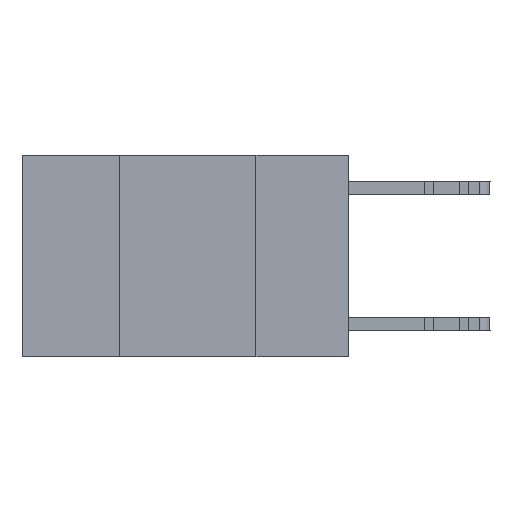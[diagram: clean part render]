
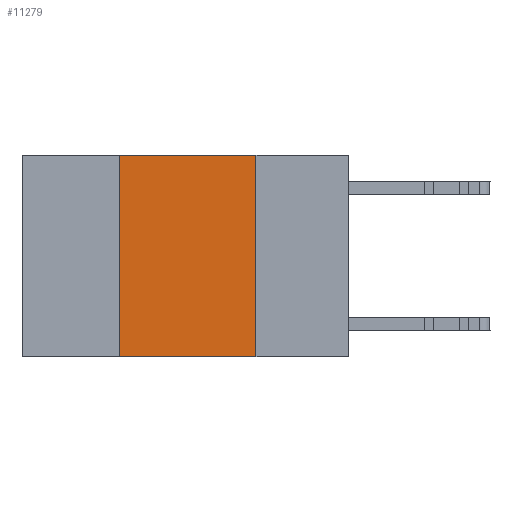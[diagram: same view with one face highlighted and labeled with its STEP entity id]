
A CAD part, left-side view. The second image highlights one B-rep face of the part: STEP entity #11279.
In plain terms, the highlighted planar face has unit normal (-1, 0, 0).
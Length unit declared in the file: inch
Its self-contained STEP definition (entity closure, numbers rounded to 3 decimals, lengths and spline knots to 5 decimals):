
#52 = AXIS2_PLACEMENT_3D ( 'NONE', #11438, #1802, #20183 ) ;
#562 = CARTESIAN_POINT ( 'NONE',  ( 0., 0.42, 0. ) ) ;
#813 = VERTEX_POINT ( 'NONE', #562 ) ;
#1142 = VERTEX_POINT ( 'NONE', #29963 ) ;
#1186 = DIRECTION ( 'NONE',  ( 0., 0., -1. ) ) ;
#1802 = DIRECTION ( 'NONE',  ( 1., 0., 0. ) ) ;
#2412 = DIRECTION ( 'NONE',  ( 0., -1., 0. ) ) ;
#3195 = LINE ( 'NONE', #12538, #23407 ) ;
#3553 = CARTESIAN_POINT ( 'NONE',  ( 0., 0.42, -0.37 ) ) ;
#8365 = LINE ( 'NONE', #12520, #25971 ) ;
#8498 = CARTESIAN_POINT ( 'NONE',  ( 0., 0.42, 0. ) ) ;
#9280 = ORIENTED_EDGE ( 'NONE', *, *, #28900, .T. ) ;
#11166 = EDGE_CURVE ( 'NONE', #21873, #1142, #8365, .T. ) ;
#11279 = ADVANCED_FACE ( 'NONE', ( #16219 ), #15923, .F. ) ;
#11438 = CARTESIAN_POINT ( 'NONE',  ( 0., 0.6, 0. ) ) ;
#12480 = EDGE_LOOP ( 'NONE', ( #18365, #25222, #22929, #9280 ) ) ;
#12520 = CARTESIAN_POINT ( 'NONE',  ( 0., 0.17, 0. ) ) ;
#12538 = CARTESIAN_POINT ( 'NONE',  ( 0., 0.6, 0. ) ) ;
#15923 = PLANE ( 'NONE',  #52 ) ;
#16219 = FACE_OUTER_BOUND ( 'NONE', #12480, .T. ) ;
#16380 = LINE ( 'NONE', #23401, #23973 ) ;
#18339 = DIRECTION ( 'NONE',  ( 0., 0., 1. ) ) ;
#18365 = ORIENTED_EDGE ( 'NONE', *, *, #11166, .F. ) ;
#20042 = CARTESIAN_POINT ( 'NONE',  ( 0., 0.17, 0. ) ) ;
#20053 = DIRECTION ( 'NONE',  ( 0., -1., 0. ) ) ;
#20183 = DIRECTION ( 'NONE',  ( 0., 0., -1. ) ) ;
#20353 = VERTEX_POINT ( 'NONE', #3553 ) ;
#21873 = VERTEX_POINT ( 'NONE', #20042 ) ;
#22319 = VECTOR ( 'NONE', #18339, 39.37008 ) ;
#22623 = EDGE_CURVE ( 'NONE', #20353, #813, #27813, .T. ) ;
#22929 = ORIENTED_EDGE ( 'NONE', *, *, #22623, .F. ) ;
#23401 = CARTESIAN_POINT ( 'NONE',  ( 0., 0.6, -0.37 ) ) ;
#23407 = VECTOR ( 'NONE', #20053, 39.37008 ) ;
#23973 = VECTOR ( 'NONE', #2412, 39.37008 ) ;
#25222 = ORIENTED_EDGE ( 'NONE', *, *, #25290, .F. ) ;
#25290 = EDGE_CURVE ( 'NONE', #813, #21873, #3195, .T. ) ;
#25971 = VECTOR ( 'NONE', #1186, 39.37008 ) ;
#27813 = LINE ( 'NONE', #8498, #22319 ) ;
#28900 = EDGE_CURVE ( 'NONE', #20353, #1142, #16380, .T. ) ;
#29963 = CARTESIAN_POINT ( 'NONE',  ( 0., 0.17, -0.37 ) ) ;
